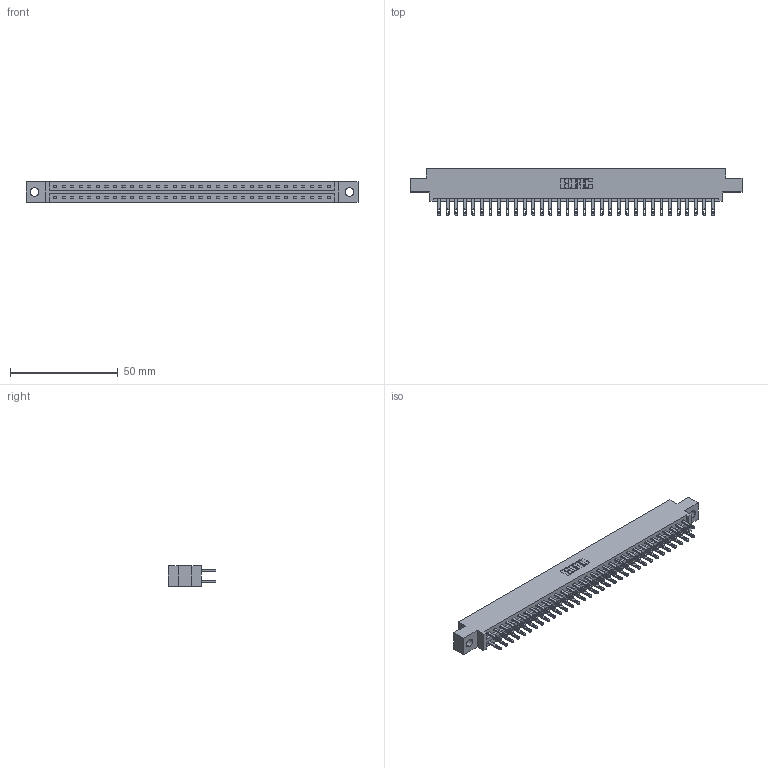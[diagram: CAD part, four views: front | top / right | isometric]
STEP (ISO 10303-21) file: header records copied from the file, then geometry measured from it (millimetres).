
FILE_DESCRIPTION (( 'STEP AP203' ), '1' );
FILE_NAME ('887-066-500-804.STEP', '2020-09-21T02:50:46', ( '' ), ( '' ), 'SwSTEP 2.0', 'SolidWorks 2020', '' );
FILE_SCHEMA (( 'CONFIG_CONTROL_DESIGN' ));
Length unit declared in the file: inch
Products named in the file (3): 345-292-001_345-293-100; 837 Part_0.170 Offset - 0.156 Dia-TH; 887-066-500-804
Assembly tree (67 placements, depth 2):
  887-066-500-804
    837 Part_0.170 Offset - 0.156 Dia-TH
    345-292-001_345-293-100  x66
Bounding box: 153.77 x 21.85 x 9.4 mm (x, y, z)
Volume: 16082.2 mm3; surface area: 18731.1 mm2
Topology: 67 solids, 67 shells, 3418 faces, 10421 edges, 6946 vertices
Faces by surface type: plane 2186, cylinder 1232
Entity records: 26815 total; most frequent: CARTESIAN_POINT 4526, ORIENTED_EDGE 4462, DIRECTION 3867, EDGE_CURVE 2231, LINE 2099, VECTOR 2099, VERTEX_POINT 1486, AXIS2_PLACEMENT_3D 884
